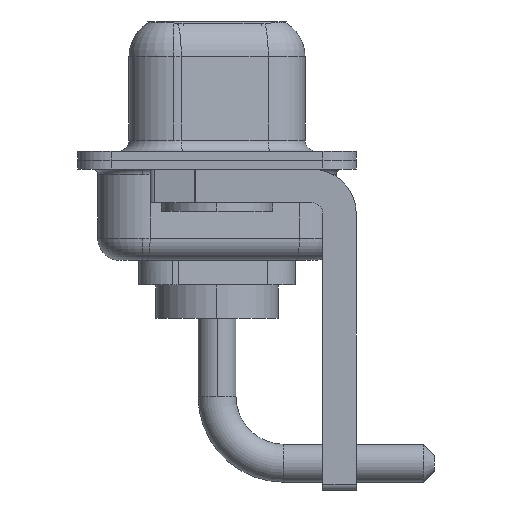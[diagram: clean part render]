
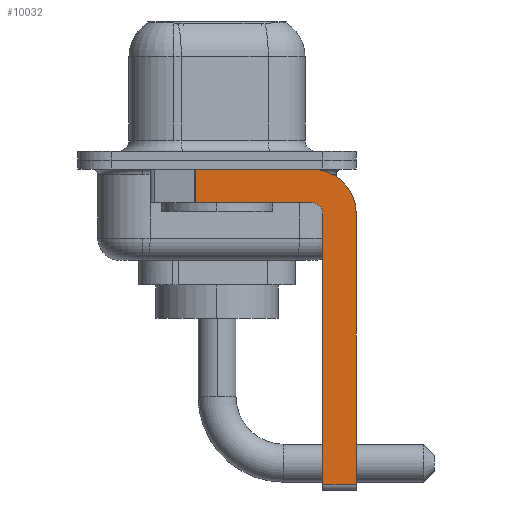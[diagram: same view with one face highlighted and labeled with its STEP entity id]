
A CAD part, left-side view. The second image highlights one B-rep face of the part: STEP entity #10032.
In plain terms, the highlighted planar face has unit normal (-1, 0, 0).
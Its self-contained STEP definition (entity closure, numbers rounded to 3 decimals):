
#591 = ORIENTED_EDGE ( 'NONE', *, *, #6087, .T. ) ;
#701 = CARTESIAN_POINT ( 'NONE',  ( -2.9, -4.25, -2.4 ) ) ;
#902 = DIRECTION ( 'NONE',  ( 0., 0., -1. ) ) ;
#959 = EDGE_CURVE ( 'NONE', #11645, #9465, #11107, .T. ) ;
#1029 = CARTESIAN_POINT ( 'NONE',  ( -2.9, 0.978, -0.4 ) ) ;
#1235 = DIRECTION ( 'NONE',  ( 0., 0., -1. ) ) ;
#1837 = EDGE_CURVE ( 'NONE', #7148, #9764, #4274, .T. ) ;
#1867 = CARTESIAN_POINT ( 'NONE',  ( -2.9, 0.978, -1.9 ) ) ;
#2285 = CARTESIAN_POINT ( 'NONE',  ( -2.9, -4.25, -0.4 ) ) ;
#2807 = EDGE_CURVE ( 'NONE', #9764, #11172, #4838, .T. ) ;
#3006 = VERTEX_POINT ( 'NONE', #5985 ) ;
#3277 = EDGE_CURVE ( 'NONE', #11172, #9465, #12330, .T. ) ;
#3367 = AXIS2_PLACEMENT_3D ( 'NONE', #10579, #12413, #7491 ) ;
#3520 = ORIENTED_EDGE ( 'NONE', *, *, #1837, .F. ) ;
#3543 = LINE ( 'NONE', #9631, #4104 ) ;
#3608 = DIRECTION ( 'NONE',  ( 0., -1., 0. ) ) ;
#3665 = CARTESIAN_POINT ( 'NONE',  ( -2.9, -6.25, -2.4 ) ) ;
#3796 = DIRECTION ( 'NONE',  ( 0., 0., -1. ) ) ;
#3906 = CARTESIAN_POINT ( 'NONE',  ( -2.9, 3., -0.4 ) ) ;
#4022 = ORIENTED_EDGE ( 'NONE', *, *, #10196, .F. ) ;
#4104 = VECTOR ( 'NONE', #3608, 1000. ) ;
#4274 = LINE ( 'NONE', #9324, #4815 ) ;
#4299 = PLANE ( 'NONE',  #11599 ) ;
#4617 = ORIENTED_EDGE ( 'NONE', *, *, #10239, .F. ) ;
#4708 = VECTOR ( 'NONE', #3796, 1000. ) ;
#4815 = VECTOR ( 'NONE', #11550, 1000. ) ;
#4838 = CIRCLE ( 'NONE', #3367, 0.5 ) ;
#5496 = CARTESIAN_POINT ( 'NONE',  ( -2.9, -6.25, -14.55 ) ) ;
#5970 = CIRCLE ( 'NONE', #10144, 2. ) ;
#5985 = CARTESIAN_POINT ( 'NONE',  ( -2.9, -6.25, -2.4 ) ) ;
#6021 = EDGE_CURVE ( 'NONE', #3006, #12675, #11725, .T. ) ;
#6087 = EDGE_CURVE ( 'NONE', #7148, #12675, #3543, .T. ) ;
#6130 = CARTESIAN_POINT ( 'NONE',  ( -2.9, 0.978, -1.9 ) ) ;
#6401 = ORIENTED_EDGE ( 'NONE', *, *, #3277, .F. ) ;
#6518 = DIRECTION ( 'NONE',  ( 1., 0., 0. ) ) ;
#6921 = DIRECTION ( 'NONE',  ( 0., -1., 0. ) ) ;
#7058 = LINE ( 'NONE', #3906, #12029 ) ;
#7148 = VERTEX_POINT ( 'NONE', #10059 ) ;
#7491 = DIRECTION ( 'NONE',  ( 0., 0., 1. ) ) ;
#7602 = CARTESIAN_POINT ( 'NONE',  ( -2.9, -4.25, -1.9 ) ) ;
#7721 = VERTEX_POINT ( 'NONE', #2285 ) ;
#8367 = CARTESIAN_POINT ( 'NONE',  ( -2.9, -4.25, -2.4 ) ) ;
#8556 = ORIENTED_EDGE ( 'NONE', *, *, #959, .T. ) ;
#8687 = DIRECTION ( 'NONE',  ( 1., 0., 0. ) ) ;
#8787 = CARTESIAN_POINT ( 'NONE',  ( -2.9, -4.25, -1.9 ) ) ;
#8986 = VECTOR ( 'NONE', #902, 1000. ) ;
#9226 = FACE_OUTER_BOUND ( 'NONE', #11714, .T. ) ;
#9324 = CARTESIAN_POINT ( 'NONE',  ( -2.9, -4.75, -14.8 ) ) ;
#9465 = VERTEX_POINT ( 'NONE', #1867 ) ;
#9631 = CARTESIAN_POINT ( 'NONE',  ( -2.9, -4.25, -14.55 ) ) ;
#9764 = VERTEX_POINT ( 'NONE', #12779 ) ;
#10032 = ADVANCED_FACE ( 'NONE', ( #9226 ), #4299, .F. ) ;
#10059 = CARTESIAN_POINT ( 'NONE',  ( -2.9, -4.75, -14.55 ) ) ;
#10128 = DIRECTION ( 'NONE',  ( 0., 0., -1. ) ) ;
#10144 = AXIS2_PLACEMENT_3D ( 'NONE', #701, #8687, #10128 ) ;
#10196 = EDGE_CURVE ( 'NONE', #7721, #3006, #5970, .T. ) ;
#10239 = EDGE_CURVE ( 'NONE', #11645, #7721, #7058, .T. ) ;
#10555 = DIRECTION ( 'NONE',  ( 0., 1., 0. ) ) ;
#10579 = CARTESIAN_POINT ( 'NONE',  ( -2.9, -4.25, -2.4 ) ) ;
#10896 = VECTOR ( 'NONE', #10555, 1000. ) ;
#11058 = ORIENTED_EDGE ( 'NONE', *, *, #2807, .F. ) ;
#11107 = LINE ( 'NONE', #6130, #8986 ) ;
#11172 = VERTEX_POINT ( 'NONE', #8787 ) ;
#11408 = ORIENTED_EDGE ( 'NONE', *, *, #6021, .F. ) ;
#11550 = DIRECTION ( 'NONE',  ( 0., 0., 1. ) ) ;
#11599 = AXIS2_PLACEMENT_3D ( 'NONE', #8367, #6518, #1235 ) ;
#11645 = VERTEX_POINT ( 'NONE', #1029 ) ;
#11714 = EDGE_LOOP ( 'NONE', ( #4617, #8556, #6401, #11058, #3520, #591, #11408, #4022 ) ) ;
#11725 = LINE ( 'NONE', #3665, #4708 ) ;
#12029 = VECTOR ( 'NONE', #6921, 1000. ) ;
#12330 = LINE ( 'NONE', #7602, #10896 ) ;
#12413 = DIRECTION ( 'NONE',  ( -1., 0., 0. ) ) ;
#12675 = VERTEX_POINT ( 'NONE', #5496 ) ;
#12779 = CARTESIAN_POINT ( 'NONE',  ( -2.9, -4.75, -2.4 ) ) ;
